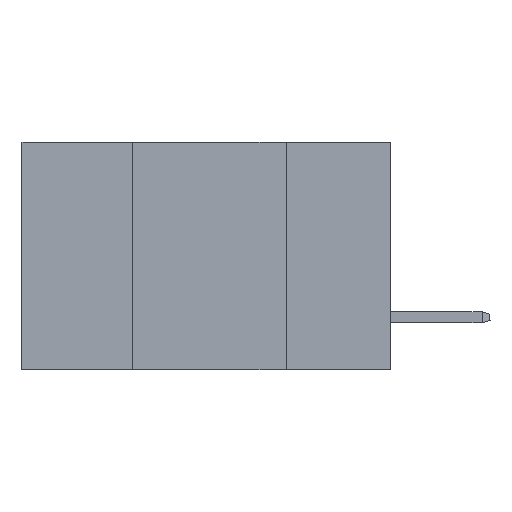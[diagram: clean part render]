
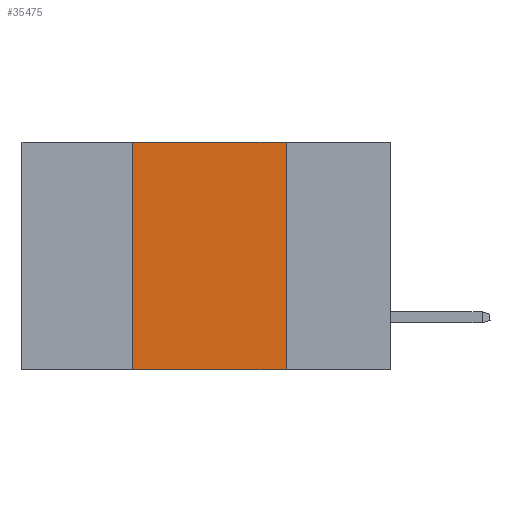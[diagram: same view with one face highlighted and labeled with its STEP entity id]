
A CAD part, left-side view. The second image highlights one B-rep face of the part: STEP entity #35475.
In plain terms, the highlighted planar face has unit normal (-1, 0, 0).
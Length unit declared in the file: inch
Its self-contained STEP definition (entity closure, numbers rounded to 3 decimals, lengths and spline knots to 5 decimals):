
#773 = CARTESIAN_POINT ( 'NONE',  ( 0., 0.17, 0. ) ) ;
#1819 = VERTEX_POINT ( 'NONE', #37017 ) ;
#2540 = EDGE_CURVE ( 'NONE', #32518, #4300, #29005, .T. ) ;
#2804 = CARTESIAN_POINT ( 'NONE',  ( 0., 0.6, -0.37 ) ) ;
#4300 = VERTEX_POINT ( 'NONE', #27045 ) ;
#4425 = CARTESIAN_POINT ( 'NONE',  ( 0., 0.6, 0. ) ) ;
#4427 = LINE ( 'NONE', #4425, #23225 ) ;
#8716 = EDGE_CURVE ( 'NONE', #13037, #1819, #31773, .T. ) ;
#9781 = DIRECTION ( 'NONE',  ( 0., -1., 0. ) ) ;
#13037 = VERTEX_POINT ( 'NONE', #773 ) ;
#16082 = AXIS2_PLACEMENT_3D ( 'NONE', #26448, #40219, #44231 ) ;
#16342 = ORIENTED_EDGE ( 'NONE', *, *, #8716, .F. ) ;
#17508 = ORIENTED_EDGE ( 'NONE', *, *, #27255, .T. ) ;
#17839 = VECTOR ( 'NONE', #30532, 39.37008 ) ;
#19230 = ORIENTED_EDGE ( 'NONE', *, *, #2540, .F. ) ;
#21569 = EDGE_CURVE ( 'NONE', #4300, #13037, #4427, .T. ) ;
#22688 = PLANE ( 'NONE',  #16082 ) ;
#22754 = LINE ( 'NONE', #2804, #25526 ) ;
#23225 = VECTOR ( 'NONE', #39845, 39.37008 ) ;
#24721 = ORIENTED_EDGE ( 'NONE', *, *, #21569, .F. ) ;
#25526 = VECTOR ( 'NONE', #9781, 39.37008 ) ;
#26448 = CARTESIAN_POINT ( 'NONE',  ( 0., 0.6, 0. ) ) ;
#26457 = DIRECTION ( 'NONE',  ( 0., 0., -1. ) ) ;
#27045 = CARTESIAN_POINT ( 'NONE',  ( 0., 0.42, 0. ) ) ;
#27255 = EDGE_CURVE ( 'NONE', #32518, #1819, #22754, .T. ) ;
#29005 = LINE ( 'NONE', #34266, #17839 ) ;
#30532 = DIRECTION ( 'NONE',  ( 0., 0., 1. ) ) ;
#30668 = VECTOR ( 'NONE', #26457, 39.37008 ) ;
#31773 = LINE ( 'NONE', #36428, #30668 ) ;
#32518 = VERTEX_POINT ( 'NONE', #33625 ) ;
#33625 = CARTESIAN_POINT ( 'NONE',  ( 0., 0.42, -0.37 ) ) ;
#34266 = CARTESIAN_POINT ( 'NONE',  ( 0., 0.42, 0. ) ) ;
#35475 = ADVANCED_FACE ( 'NONE', ( #43866 ), #22688, .F. ) ;
#36428 = CARTESIAN_POINT ( 'NONE',  ( 0., 0.17, 0. ) ) ;
#37017 = CARTESIAN_POINT ( 'NONE',  ( 0., 0.17, -0.37 ) ) ;
#39845 = DIRECTION ( 'NONE',  ( 0., -1., 0. ) ) ;
#40219 = DIRECTION ( 'NONE',  ( 1., 0., 0. ) ) ;
#42607 = EDGE_LOOP ( 'NONE', ( #16342, #24721, #19230, #17508 ) ) ;
#43866 = FACE_OUTER_BOUND ( 'NONE', #42607, .T. ) ;
#44231 = DIRECTION ( 'NONE',  ( 0., 0., -1. ) ) ;
